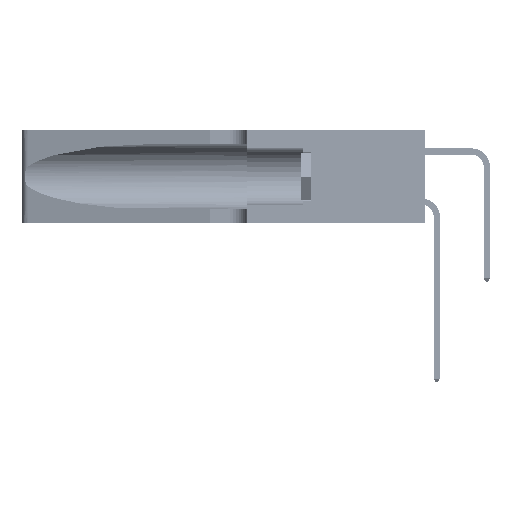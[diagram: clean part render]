
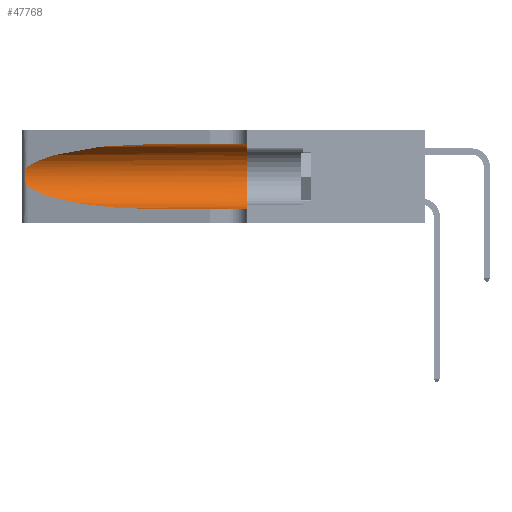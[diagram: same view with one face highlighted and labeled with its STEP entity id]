
A CAD part, left-side view. The second image highlights one B-rep face of the part: STEP entity #47768.
In plain terms, the highlighted cylindrical face has radius 3.308 mm (diameter 6.617 mm), a partial arc.
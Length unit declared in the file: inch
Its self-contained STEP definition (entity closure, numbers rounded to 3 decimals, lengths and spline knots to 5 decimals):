
#19 = EDGE_CURVE ( 'NONE', #1340, #2891, #19692, .T. ) ;
#1340 = VERTEX_POINT ( 'NONE', #15118 ) ;
#1493 = CARTESIAN_POINT ( 'NONE',  ( 0.25487, 1.22718, 0.14631 ) ) ;
#2005 = CARTESIAN_POINT ( 'NONE',  ( 0.18966, 0.96281, 0.05475 ) ) ;
#2019 = DIRECTION ( 'NONE',  ( 0., -1., 0. ) ) ;
#2194 =( BOUNDED_CURVE ( )  B_SPLINE_CURVE ( 3, ( #3806, #31898, #12053, #40320 ),
 .UNSPECIFIED., .F., .T. ) 
 B_SPLINE_CURVE_WITH_KNOTS ( ( 4, 4 ),
 ( 1.5708, 2.84003 ),
 .UNSPECIFIED. ) 
 CURVE ( )  GEOMETRIC_REPRESENTATION_ITEM ( )  RATIONAL_B_SPLINE_CURVE ( ( 1., 0.87, 0.87, 1. ) ) 
 REPRESENTATION_ITEM ( '' )  );
#2734 = DIRECTION ( 'NONE',  ( 0., 0., 1. ) ) ;
#2891 = VERTEX_POINT ( 'NONE', #7873 ) ;
#3806 = CARTESIAN_POINT ( 'NONE',  ( 0.1305, 0.72297, 0.31525 ) ) ;
#4834 = CARTESIAN_POINT ( 'NONE',  ( 0.25487, 1.22718, 0.22369 ) ) ;
#5446 = CARTESIAN_POINT ( 'NONE',  ( 0.25639, 1.23184, 0.21858 ) ) ;
#6913 = ORIENTED_EDGE ( 'NONE', *, *, #32937, .F. ) ;
#7409 = AXIS2_PLACEMENT_3D ( 'NONE', #41213, #20917, #24978 ) ;
#7857 =( BOUNDED_CURVE ( )  B_SPLINE_CURVE ( 3, ( #26703, #22650, #2005, #30791 ),
 .UNSPECIFIED., .F., .F. ) 
 B_SPLINE_CURVE_WITH_KNOTS ( ( 4, 4 ),
 ( 3.44316, 4.71239 ),
 .UNSPECIFIED. ) 
 CURVE ( )  GEOMETRIC_REPRESENTATION_ITEM ( )  RATIONAL_B_SPLINE_CURVE ( ( 1., 0.87, 0.87, 1. ) ) 
 REPRESENTATION_ITEM ( '' )  );
#7873 = CARTESIAN_POINT ( 'NONE',  ( 0.1305, 0.35, 0.31525 ) ) ;
#9565 = CARTESIAN_POINT ( 'NONE',  ( 0.25854, 1.2359, 0.20912 ) ) ;
#12053 = CARTESIAN_POINT ( 'NONE',  ( 0.2373, 1.15595, 0.28018 ) ) ;
#13672 = CARTESIAN_POINT ( 'NONE',  ( 0.26075, 1.23896, 0.19203 ) ) ;
#15118 = CARTESIAN_POINT ( 'NONE',  ( 0.1305, 0.72297, 0.31525 ) ) ;
#16232 = EDGE_CURVE ( 'NONE', #27482, #33117, #7857, .T. ) ;
#17653 = ORIENTED_EDGE ( 'NONE', *, *, #31122, .T. ) ;
#17735 = CARTESIAN_POINT ( 'NONE',  ( 0.26017, 1.23833, 0.17102 ) ) ;
#19692 = LINE ( 'NONE', #50551, #30440 ) ;
#20917 = DIRECTION ( 'NONE',  ( 0., -1., 0. ) ) ;
#21815 = CARTESIAN_POINT ( 'NONE',  ( 0.25789, 1.23486, 0.15765 ) ) ;
#21893 = VERTEX_POINT ( 'NONE', #34232 ) ;
#22650 = CARTESIAN_POINT ( 'NONE',  ( 0.2373, 1.15595, 0.08982 ) ) ;
#23258 = DIRECTION ( 'NONE',  ( 0., -1., 0. ) ) ;
#24978 = DIRECTION ( 'NONE',  ( 0., 0., -1. ) ) ;
#25687 = CARTESIAN_POINT ( 'NONE',  ( 0.25487, 1.22718, 0.22369 ) ) ;
#25857 = CARTESIAN_POINT ( 'NONE',  ( 0.25555, 1.22993, 0.14849 ) ) ;
#26090 = CIRCLE ( 'NONE', #31816, 0.13025 ) ;
#26703 = CARTESIAN_POINT ( 'NONE',  ( 0.25487, 1.22718, 0.14631 ) ) ;
#27094 = DIRECTION ( 'NONE',  ( 0., 1., 0. ) ) ;
#27428 = EDGE_LOOP ( 'NONE', ( #17653, #39583, #47683, #50993, #6913, #47744 ) ) ;
#27482 = VERTEX_POINT ( 'NONE', #40865 ) ;
#30063 = EDGE_CURVE ( 'NONE', #33117, #21893, #48613, .T. ) ;
#30440 = VECTOR ( 'NONE', #2019, 39.37008 ) ;
#30791 = CARTESIAN_POINT ( 'NONE',  ( 0.1305, 0.72297, 0.05475 ) ) ;
#31122 = EDGE_CURVE ( 'NONE', #1340, #38412, #2194, .T. ) ;
#31816 = AXIS2_PLACEMENT_3D ( 'NONE', #51253, #27094, #2734 ) ;
#31898 = CARTESIAN_POINT ( 'NONE',  ( 0.18966, 0.96281, 0.31525 ) ) ;
#32491 = CYLINDRICAL_SURFACE ( 'NONE', #7409, 0.13025 ) ;
#32937 = EDGE_CURVE ( 'NONE', #2891, #21893, #26090, .T. ) ;
#33117 = VERTEX_POINT ( 'NONE', #44182 ) ;
#33755 = FACE_OUTER_BOUND ( 'NONE', #27428, .T. ) ;
#33851 = CARTESIAN_POINT ( 'NONE',  ( 0.25787, 1.23484, 0.2124 ) ) ;
#34232 = CARTESIAN_POINT ( 'NONE',  ( 0.1305, 0.35, 0.05475 ) ) ;
#36606 = VECTOR ( 'NONE', #23258, 39.37008 ) ;
#37875 = CARTESIAN_POINT ( 'NONE',  ( 0.26018, 1.23835, 0.19895 ) ) ;
#38412 = VERTEX_POINT ( 'NONE', #4834 ) ;
#39583 = ORIENTED_EDGE ( 'NONE', *, *, #51702, .T. ) ;
#40320 = CARTESIAN_POINT ( 'NONE',  ( 0.25487, 1.22718, 0.22369 ) ) ;
#40865 = CARTESIAN_POINT ( 'NONE',  ( 0.25487, 1.22718, 0.14631 ) ) ;
#41213 = CARTESIAN_POINT ( 'NONE',  ( 0.1305, 1.61858, 0.185 ) ) ;
#41918 = CARTESIAN_POINT ( 'NONE',  ( 0.26075, 1.23896, 0.178 ) ) ;
#44182 = CARTESIAN_POINT ( 'NONE',  ( 0.1305, 0.72297, 0.05475 ) ) ;
#45994 = CARTESIAN_POINT ( 'NONE',  ( 0.25856, 1.23593, 0.16098 ) ) ;
#47446 = CARTESIAN_POINT ( 'NONE',  ( 0.1305, 1.61858, 0.05475 ) ) ;
#47683 = ORIENTED_EDGE ( 'NONE', *, *, #16232, .T. ) ;
#47744 = ORIENTED_EDGE ( 'NONE', *, *, #19, .F. ) ;
#47768 = ADVANCED_FACE ( 'NONE', ( #33755 ), #32491, .F. ) ;
#48613 = LINE ( 'NONE', #47446, #36606 ) ;
#49858 = CARTESIAN_POINT ( 'NONE',  ( 0.25555, 1.22994, 0.2215 ) ) ;
#50037 = CARTESIAN_POINT ( 'NONE',  ( 0.25639, 1.23186, 0.15144 ) ) ;
#50551 = CARTESIAN_POINT ( 'NONE',  ( 0.1305, 1.61858, 0.31525 ) ) ;
#50993 = ORIENTED_EDGE ( 'NONE', *, *, #30063, .T. ) ;
#51253 = CARTESIAN_POINT ( 'NONE',  ( 0.1305, 0.35, 0.185 ) ) ;
#51616 = B_SPLINE_CURVE_WITH_KNOTS ( 'NONE', 3,
 ( #25687, #49858, #5446, #33851, #9565, #37875, #13672, #41918, #17735, #45994, #21815, #50037, #25857, #1493 ),
 .UNSPECIFIED., .F., .F.,
 ( 4, 2, 2, 2, 2, 2, 4 ),
 ( 0., 0.00027, 0.00053, 0.00107, 0.0016, 0.00187, 0.00214 ),
 .UNSPECIFIED. ) ;
#51702 = EDGE_CURVE ( 'NONE', #38412, #27482, #51616, .T. ) ;
